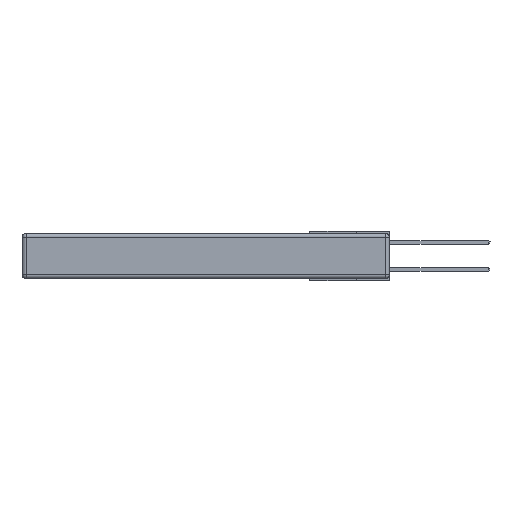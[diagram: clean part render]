
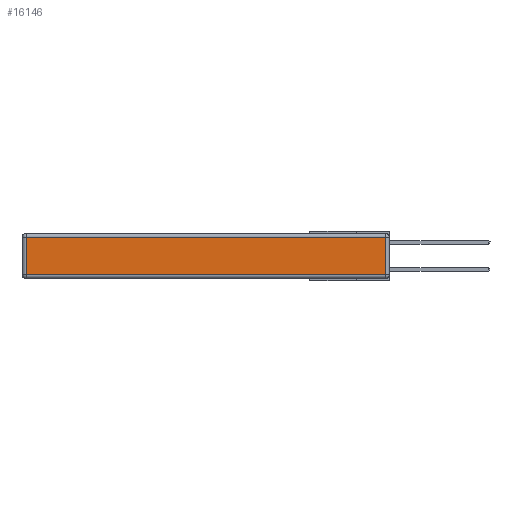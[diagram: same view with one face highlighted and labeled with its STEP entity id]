
A CAD part, left-side view. The second image highlights one B-rep face of the part: STEP entity #16146.
In plain terms, the highlighted planar face has unit normal (-1, 0, 0).
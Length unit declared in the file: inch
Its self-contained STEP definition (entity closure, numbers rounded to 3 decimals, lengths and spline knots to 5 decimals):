
#792 = CARTESIAN_POINT ( 'NONE',  ( 0., 0.03, -0.343 ) ) ;
#1948 = VERTEX_POINT ( 'NONE', #14008 ) ;
#2499 = ORIENTED_EDGE ( 'NONE', *, *, #14483, .T. ) ;
#4078 = LINE ( 'NONE', #10022, #21479 ) ;
#4159 = ORIENTED_EDGE ( 'NONE', *, *, #17302, .T. ) ;
#4574 = CARTESIAN_POINT ( 'NONE',  ( 0., 0.03, -0.03 ) ) ;
#5746 = FACE_OUTER_BOUND ( 'NONE', #13046, .T. ) ;
#5871 = DIRECTION ( 'NONE',  ( 0., 0., 1. ) ) ;
#6274 = AXIS2_PLACEMENT_3D ( 'NONE', #9719, #7834, #11266 ) ;
#6781 = LINE ( 'NONE', #792, #19662 ) ;
#7834 = DIRECTION ( 'NONE',  ( -1., 0., 0. ) ) ;
#8139 = PLANE ( 'NONE',  #6274 ) ;
#8153 = CARTESIAN_POINT ( 'NONE',  ( 0., 2.72, -0.343 ) ) ;
#9719 = CARTESIAN_POINT ( 'NONE',  ( 0., 0., -0.343 ) ) ;
#10022 = CARTESIAN_POINT ( 'NONE',  ( 0., 0., -0.313 ) ) ;
#10307 = LINE ( 'NONE', #8153, #12635 ) ;
#10338 = EDGE_CURVE ( 'NONE', #15884, #11267, #10307, .T. ) ;
#11266 = DIRECTION ( 'NONE',  ( 0., 0., 1. ) ) ;
#11267 = VERTEX_POINT ( 'NONE', #19168 ) ;
#11268 = ORIENTED_EDGE ( 'NONE', *, *, #16434, .T. ) ;
#11744 = DIRECTION ( 'NONE',  ( 0., 0., -1. ) ) ;
#12287 = CARTESIAN_POINT ( 'NONE',  ( 0., 2.72, -0.03 ) ) ;
#12461 = CARTESIAN_POINT ( 'NONE',  ( 0., 2.75, -0.03 ) ) ;
#12635 = VECTOR ( 'NONE', #11744, 39.37008 ) ;
#13046 = EDGE_LOOP ( 'NONE', ( #2499, #4159, #11268, #21310 ) ) ;
#14008 = CARTESIAN_POINT ( 'NONE',  ( 0., 0.03, -0.313 ) ) ;
#14483 = EDGE_CURVE ( 'NONE', #11267, #1948, #4078, .T. ) ;
#15884 = VERTEX_POINT ( 'NONE', #12287 ) ;
#16146 = ADVANCED_FACE ( 'NONE', ( #5746 ), #8139, .T. ) ;
#16434 = EDGE_CURVE ( 'NONE', #19697, #15884, #21769, .T. ) ;
#17231 = DIRECTION ( 'NONE',  ( 0., 1., 0. ) ) ;
#17302 = EDGE_CURVE ( 'NONE', #1948, #19697, #6781, .T. ) ;
#17836 = VECTOR ( 'NONE', #17231, 39.37008 ) ;
#19168 = CARTESIAN_POINT ( 'NONE',  ( 0., 2.72, -0.313 ) ) ;
#19662 = VECTOR ( 'NONE', #5871, 39.37008 ) ;
#19697 = VERTEX_POINT ( 'NONE', #4574 ) ;
#21310 = ORIENTED_EDGE ( 'NONE', *, *, #10338, .T. ) ;
#21479 = VECTOR ( 'NONE', #21724, 39.37008 ) ;
#21724 = DIRECTION ( 'NONE',  ( 0., -1., 0. ) ) ;
#21769 = LINE ( 'NONE', #12461, #17836 ) ;
